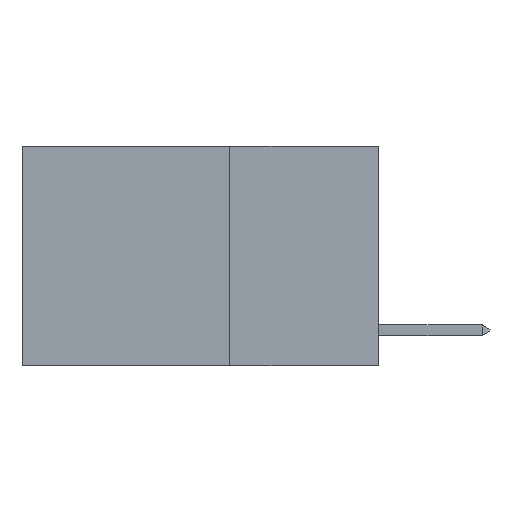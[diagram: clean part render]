
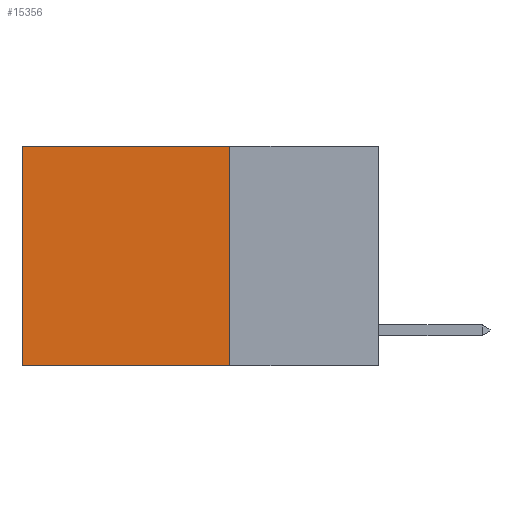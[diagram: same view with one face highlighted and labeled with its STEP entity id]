
A CAD part, left-side view. The second image highlights one B-rep face of the part: STEP entity #15356.
In plain terms, the highlighted planar face has unit normal (-1, 0, 0).
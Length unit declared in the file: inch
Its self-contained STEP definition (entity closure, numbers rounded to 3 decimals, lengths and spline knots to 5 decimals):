
#354 = AXIS2_PLACEMENT_3D ( 'NONE', #15980, #9382, #1435 ) ;
#440 = LINE ( 'NONE', #4945, #11639 ) ;
#716 = LINE ( 'NONE', #16083, #14638 ) ;
#1063 = FACE_OUTER_BOUND ( 'NONE', #13806, .T. ) ;
#1435 = DIRECTION ( 'NONE',  ( 0., 0., -1. ) ) ;
#2284 = ORIENTED_EDGE ( 'NONE', *, *, #11713, .T. ) ;
#3133 = CARTESIAN_POINT ( 'NONE',  ( 0.2625, 0.25, -0.37 ) ) ;
#3318 = CARTESIAN_POINT ( 'NONE',  ( 0.2625, 0.6, -0.37 ) ) ;
#3429 = VERTEX_POINT ( 'NONE', #3318 ) ;
#4052 = CARTESIAN_POINT ( 'NONE',  ( 0.2625, 0.25, 0. ) ) ;
#4945 = CARTESIAN_POINT ( 'NONE',  ( 0.2625, 0.25, 0. ) ) ;
#5381 = VERTEX_POINT ( 'NONE', #8908 ) ;
#5686 = LINE ( 'NONE', #14087, #10235 ) ;
#5817 = ORIENTED_EDGE ( 'NONE', *, *, #7520, .T. ) ;
#6707 = DIRECTION ( 'NONE',  ( 0., 0., -1. ) ) ;
#7520 = EDGE_CURVE ( 'NONE', #12416, #5381, #7933, .T. ) ;
#7933 = LINE ( 'NONE', #10904, #12705 ) ;
#8084 = DIRECTION ( 'NONE',  ( 0., 1., 0. ) ) ;
#8908 = CARTESIAN_POINT ( 'NONE',  ( 0.2625, 0.6, 0. ) ) ;
#9382 = DIRECTION ( 'NONE',  ( 1., 0., 0. ) ) ;
#10235 = VECTOR ( 'NONE', #11458, 39.37008 ) ;
#10904 = CARTESIAN_POINT ( 'NONE',  ( 0.2625, 0.25, 0. ) ) ;
#11362 = ORIENTED_EDGE ( 'NONE', *, *, #14689, .F. ) ;
#11458 = DIRECTION ( 'NONE',  ( 0., 1., 0. ) ) ;
#11639 = VECTOR ( 'NONE', #11721, 39.37008 ) ;
#11713 = EDGE_CURVE ( 'NONE', #5381, #3429, #716, .T. ) ;
#11721 = DIRECTION ( 'NONE',  ( 0., 0., -1. ) ) ;
#12101 = EDGE_CURVE ( 'NONE', #15040, #3429, #5686, .T. ) ;
#12416 = VERTEX_POINT ( 'NONE', #4052 ) ;
#12705 = VECTOR ( 'NONE', #8084, 39.37008 ) ;
#13352 = PLANE ( 'NONE',  #354 ) ;
#13806 = EDGE_LOOP ( 'NONE', ( #2284, #17013, #11362, #5817 ) ) ;
#14087 = CARTESIAN_POINT ( 'NONE',  ( 0.2625, 0.25, -0.37 ) ) ;
#14638 = VECTOR ( 'NONE', #6707, 39.37008 ) ;
#14689 = EDGE_CURVE ( 'NONE', #12416, #15040, #440, .T. ) ;
#15040 = VERTEX_POINT ( 'NONE', #3133 ) ;
#15356 = ADVANCED_FACE ( 'NONE', ( #1063 ), #13352, .F. ) ;
#15980 = CARTESIAN_POINT ( 'NONE',  ( 0.2625, 0.25, 0. ) ) ;
#16083 = CARTESIAN_POINT ( 'NONE',  ( 0.2625, 0.6, 0. ) ) ;
#17013 = ORIENTED_EDGE ( 'NONE', *, *, #12101, .F. ) ;
